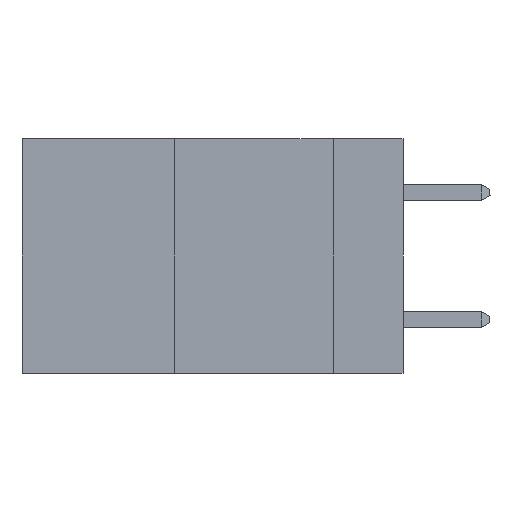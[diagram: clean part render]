
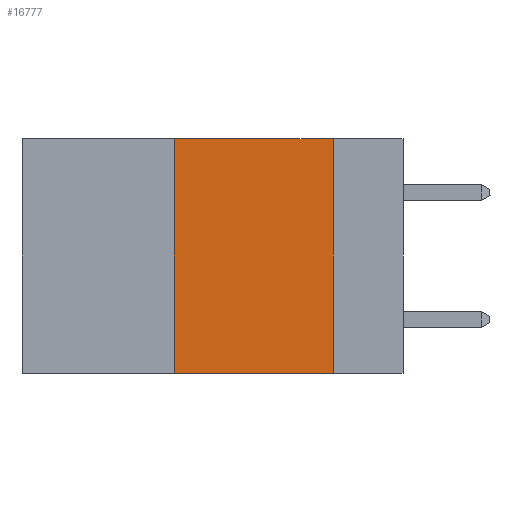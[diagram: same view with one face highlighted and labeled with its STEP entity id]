
A CAD part, left-side view. The second image highlights one B-rep face of the part: STEP entity #16777.
In plain terms, the highlighted planar face has unit normal (-1, 0, 0).
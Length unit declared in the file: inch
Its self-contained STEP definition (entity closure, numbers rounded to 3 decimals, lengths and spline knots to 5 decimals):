
#47 = DIRECTION ( 'NONE',  ( 0., -1., 0. ) ) ;
#537 = ORIENTED_EDGE ( 'NONE', *, *, #12083, .T. ) ;
#1143 = VERTEX_POINT ( 'NONE', #19748 ) ;
#1752 = VERTEX_POINT ( 'NONE', #25832 ) ;
#4006 = LINE ( 'NONE', #14976, #30286 ) ;
#5219 = CARTESIAN_POINT ( 'NONE',  ( 0., 0.36, -0.37 ) ) ;
#5280 = DIRECTION ( 'NONE',  ( 1., 0., 0. ) ) ;
#5332 = EDGE_LOOP ( 'NONE', ( #9960, #13984, #8930, #537 ) ) ;
#5333 = CARTESIAN_POINT ( 'NONE',  ( 0., 0.6, 0. ) ) ;
#8296 = FACE_OUTER_BOUND ( 'NONE', #5332, .T. ) ;
#8930 = ORIENTED_EDGE ( 'NONE', *, *, #24398, .F. ) ;
#9960 = ORIENTED_EDGE ( 'NONE', *, *, #34068, .F. ) ;
#12083 = EDGE_CURVE ( 'NONE', #23051, #1143, #4006, .T. ) ;
#13878 = VECTOR ( 'NONE', #47, 39.37008 ) ;
#13984 = ORIENTED_EDGE ( 'NONE', *, *, #33715, .F. ) ;
#14113 = CARTESIAN_POINT ( 'NONE',  ( 0., 0.11, 0. ) ) ;
#14976 = CARTESIAN_POINT ( 'NONE',  ( 0., 0.6, -0.37 ) ) ;
#16568 = PLANE ( 'NONE',  #16918 ) ;
#16777 = ADVANCED_FACE ( 'NONE', ( #8296 ), #16568, .F. ) ;
#16918 = AXIS2_PLACEMENT_3D ( 'NONE', #22219, #5280, #24874 ) ;
#19748 = CARTESIAN_POINT ( 'NONE',  ( 0., 0.11, -0.37 ) ) ;
#20148 = CARTESIAN_POINT ( 'NONE',  ( 0., 0.36, 0. ) ) ;
#20459 = CARTESIAN_POINT ( 'NONE',  ( 0., 0.36, 0. ) ) ;
#21400 = LINE ( 'NONE', #5333, #13878 ) ;
#21724 = VECTOR ( 'NONE', #34212, 39.37008 ) ;
#21884 = DIRECTION ( 'NONE',  ( 0., 0., -1. ) ) ;
#22219 = CARTESIAN_POINT ( 'NONE',  ( 0., 0.6, 0. ) ) ;
#23051 = VERTEX_POINT ( 'NONE', #5219 ) ;
#23076 = DIRECTION ( 'NONE',  ( 0., -1., 0. ) ) ;
#23459 = VECTOR ( 'NONE', #21884, 39.37008 ) ;
#24398 = EDGE_CURVE ( 'NONE', #23051, #27368, #28760, .T. ) ;
#24874 = DIRECTION ( 'NONE',  ( 0., 0., -1. ) ) ;
#25832 = CARTESIAN_POINT ( 'NONE',  ( 0., 0.11, 0. ) ) ;
#27368 = VERTEX_POINT ( 'NONE', #20148 ) ;
#28760 = LINE ( 'NONE', #20459, #21724 ) ;
#30165 = LINE ( 'NONE', #14113, #23459 ) ;
#30286 = VECTOR ( 'NONE', #23076, 39.37008 ) ;
#33715 = EDGE_CURVE ( 'NONE', #27368, #1752, #21400, .T. ) ;
#34068 = EDGE_CURVE ( 'NONE', #1752, #1143, #30165, .T. ) ;
#34212 = DIRECTION ( 'NONE',  ( 0., 0., 1. ) ) ;
